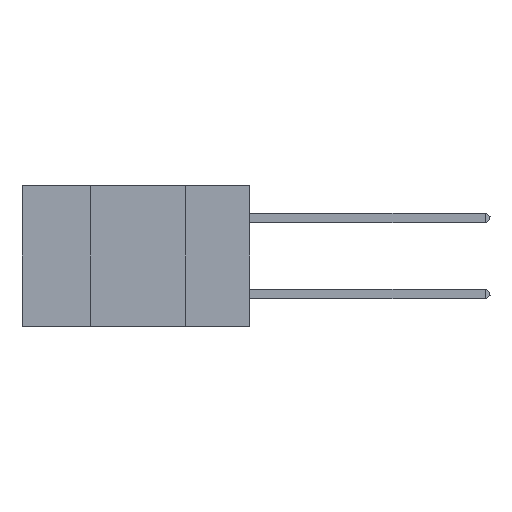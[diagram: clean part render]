
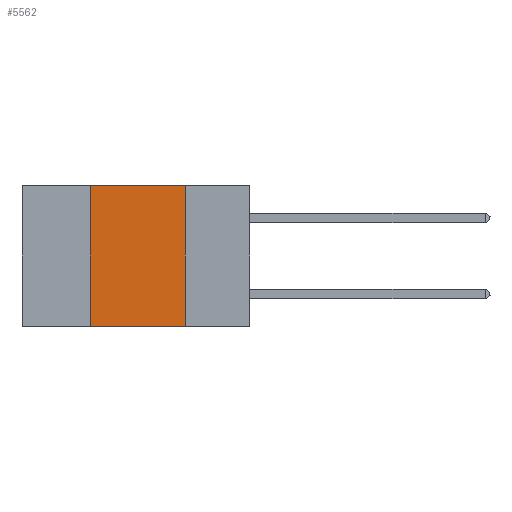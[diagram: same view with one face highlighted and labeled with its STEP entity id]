
A CAD part, left-side view. The second image highlights one B-rep face of the part: STEP entity #5562.
In plain terms, the highlighted planar face has unit normal (-1, 0, 0).
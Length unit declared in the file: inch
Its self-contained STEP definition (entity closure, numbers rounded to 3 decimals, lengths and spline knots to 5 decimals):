
#265 = ORIENTED_EDGE ( 'NONE', *, *, #3945, .F. ) ;
#331 = ORIENTED_EDGE ( 'NONE', *, *, #17850, .F. ) ;
#2154 = ORIENTED_EDGE ( 'NONE', *, *, #33260, .F. ) ;
#3736 = ORIENTED_EDGE ( 'NONE', *, *, #13510, .T. ) ;
#3945 = EDGE_CURVE ( 'NONE', #7233, #11418, #16129, .T. ) ;
#4565 = DIRECTION ( 'NONE',  ( 1., 0., 0. ) ) ;
#5562 = ADVANCED_FACE ( 'NONE', ( #26608 ), #32876, .F. ) ;
#5732 = CARTESIAN_POINT ( 'NONE',  ( 0., 0.17, -0.37 ) ) ;
#7233 = VERTEX_POINT ( 'NONE', #32246 ) ;
#7606 = CARTESIAN_POINT ( 'NONE',  ( 0., 0.17, 0. ) ) ;
#8415 = VECTOR ( 'NONE', #20650, 39.37008 ) ;
#10527 = CARTESIAN_POINT ( 'NONE',  ( 0., 0.6, -0.37 ) ) ;
#10648 = DIRECTION ( 'NONE',  ( 0., -1., 0. ) ) ;
#11258 = VECTOR ( 'NONE', #10648, 39.37008 ) ;
#11418 = VERTEX_POINT ( 'NONE', #20847 ) ;
#11474 = DIRECTION ( 'NONE',  ( 0., -1., 0. ) ) ;
#13510 = EDGE_CURVE ( 'NONE', #7233, #16581, #24995, .T. ) ;
#14057 = DIRECTION ( 'NONE',  ( 0., 0., 1. ) ) ;
#15230 = AXIS2_PLACEMENT_3D ( 'NONE', #20317, #4565, #22831 ) ;
#15865 = EDGE_LOOP ( 'NONE', ( #2154, #331, #265, #3736 ) ) ;
#16129 = LINE ( 'NONE', #29381, #22915 ) ;
#16581 = VERTEX_POINT ( 'NONE', #5732 ) ;
#16775 = CARTESIAN_POINT ( 'NONE',  ( 0., 0.6, 0. ) ) ;
#17850 = EDGE_CURVE ( 'NONE', #11418, #27180, #20188, .T. ) ;
#20188 = LINE ( 'NONE', #16775, #26932 ) ;
#20317 = CARTESIAN_POINT ( 'NONE',  ( 0., 0.6, 0. ) ) ;
#20650 = DIRECTION ( 'NONE',  ( 0., 0., -1. ) ) ;
#20847 = CARTESIAN_POINT ( 'NONE',  ( 0., 0.42, 0. ) ) ;
#22831 = DIRECTION ( 'NONE',  ( 0., 0., -1. ) ) ;
#22915 = VECTOR ( 'NONE', #14057, 39.37008 ) ;
#23409 = CARTESIAN_POINT ( 'NONE',  ( 0., 0.17, 0. ) ) ;
#24995 = LINE ( 'NONE', #10527, #11258 ) ;
#26608 = FACE_OUTER_BOUND ( 'NONE', #15865, .T. ) ;
#26932 = VECTOR ( 'NONE', #11474, 39.37008 ) ;
#27180 = VERTEX_POINT ( 'NONE', #23409 ) ;
#29381 = CARTESIAN_POINT ( 'NONE',  ( 0., 0.42, 0. ) ) ;
#29809 = LINE ( 'NONE', #7606, #8415 ) ;
#32246 = CARTESIAN_POINT ( 'NONE',  ( 0., 0.42, -0.37 ) ) ;
#32876 = PLANE ( 'NONE',  #15230 ) ;
#33260 = EDGE_CURVE ( 'NONE', #27180, #16581, #29809, .T. ) ;
